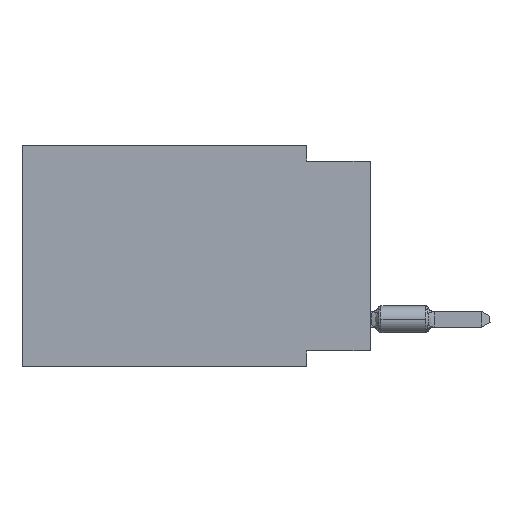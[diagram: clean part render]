
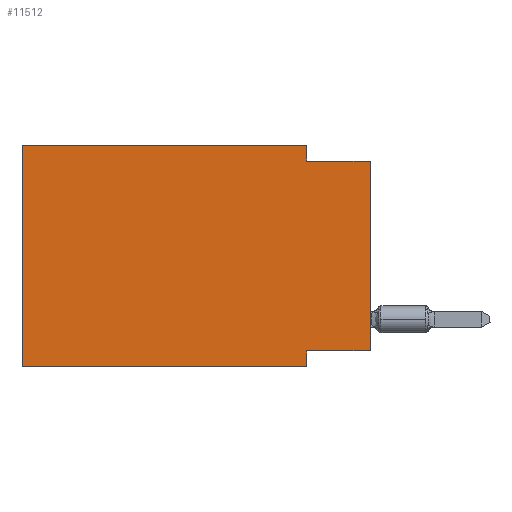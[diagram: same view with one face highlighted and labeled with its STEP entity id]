
A CAD part, left-side view. The second image highlights one B-rep face of the part: STEP entity #11512.
In plain terms, the highlighted planar face has unit normal (-1, 0, 0).
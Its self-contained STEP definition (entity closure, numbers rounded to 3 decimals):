
#978 = ORIENTED_EDGE ( 'NONE', *, *, #32327, .F. ) ;
#1175 = DIRECTION ( 'NONE',  ( 0., 0., -1. ) ) ;
#1207 = CARTESIAN_POINT ( 'NONE',  ( 0., 0., -8.255 ) ) ;
#1449 = CARTESIAN_POINT ( 'NONE',  ( 0., 0., -0.635 ) ) ;
#2517 = CARTESIAN_POINT ( 'NONE',  ( 0., 2.54, -8.255 ) ) ;
#3045 = ORIENTED_EDGE ( 'NONE', *, *, #33190, .F. ) ;
#3414 = VECTOR ( 'NONE', #35923, 1000. ) ;
#5371 = CARTESIAN_POINT ( 'NONE',  ( 0., 13.97, -8.89 ) ) ;
#5551 = EDGE_LOOP ( 'NONE', ( #31347, #14527, #7653, #40815, #9410, #18989, #3045, #978 ) ) ;
#5599 = EDGE_CURVE ( 'NONE', #5946, #6563, #39292, .T. ) ;
#5946 = VERTEX_POINT ( 'NONE', #5371 ) ;
#6563 = VERTEX_POINT ( 'NONE', #30222 ) ;
#6693 = CARTESIAN_POINT ( 'NONE',  ( 0., 13.97, 0. ) ) ;
#7653 = ORIENTED_EDGE ( 'NONE', *, *, #34721, .F. ) ;
#8140 = EDGE_CURVE ( 'NONE', #22937, #24792, #32397, .T. ) ;
#8572 = VECTOR ( 'NONE', #19413, 1000. ) ;
#9410 = ORIENTED_EDGE ( 'NONE', *, *, #16517, .F. ) ;
#9543 = CARTESIAN_POINT ( 'NONE',  ( 0., 13.97, 0. ) ) ;
#9876 = VECTOR ( 'NONE', #12463, 1000. ) ;
#10045 = DIRECTION ( 'NONE',  ( 1., 0., 0. ) ) ;
#10299 = CARTESIAN_POINT ( 'NONE',  ( 0., 2.54, -0.635 ) ) ;
#10809 = CARTESIAN_POINT ( 'NONE',  ( 0., 2.54, 0. ) ) ;
#11512 = ADVANCED_FACE ( 'NONE', ( #43934 ), #30256, .F. ) ;
#11811 = EDGE_CURVE ( 'NONE', #14311, #24792, #18975, .T. ) ;
#12463 = DIRECTION ( 'NONE',  ( 0., -1., 0. ) ) ;
#13838 = EDGE_CURVE ( 'NONE', #37819, #35714, #14929, .T. ) ;
#14311 = VERTEX_POINT ( 'NONE', #1207 ) ;
#14527 = ORIENTED_EDGE ( 'NONE', *, *, #8140, .F. ) ;
#14922 = VECTOR ( 'NONE', #15332, 1000. ) ;
#14929 = LINE ( 'NONE', #38952, #9876 ) ;
#15220 = LINE ( 'NONE', #39028, #25471 ) ;
#15332 = DIRECTION ( 'NONE',  ( 0., -1., 0. ) ) ;
#16517 = EDGE_CURVE ( 'NONE', #5946, #37819, #37134, .T. ) ;
#18211 = LINE ( 'NONE', #39086, #34447 ) ;
#18518 = DIRECTION ( 'NONE',  ( 0., 0., 1. ) ) ;
#18975 = LINE ( 'NONE', #22107, #25456 ) ;
#18989 = ORIENTED_EDGE ( 'NONE', *, *, #5599, .T. ) ;
#19413 = DIRECTION ( 'NONE',  ( 0., 0., 1. ) ) ;
#19772 = CARTESIAN_POINT ( 'NONE',  ( 0., 0., -0.635 ) ) ;
#20135 = DIRECTION ( 'NONE',  ( 0., 0., -1. ) ) ;
#22107 = CARTESIAN_POINT ( 'NONE',  ( 0., 0., 0. ) ) ;
#22451 = CARTESIAN_POINT ( 'NONE',  ( 0., 13.97, -8.89 ) ) ;
#22937 = VERTEX_POINT ( 'NONE', #10299 ) ;
#24792 = VERTEX_POINT ( 'NONE', #19772 ) ;
#25456 = VECTOR ( 'NONE', #18518, 1000. ) ;
#25471 = VECTOR ( 'NONE', #38584, 1000. ) ;
#26122 = VERTEX_POINT ( 'NONE', #2517 ) ;
#29053 = AXIS2_PLACEMENT_3D ( 'NONE', #6693, #10045, #34266 ) ;
#30222 = CARTESIAN_POINT ( 'NONE',  ( 0., 2.54, -8.89 ) ) ;
#30256 = PLANE ( 'NONE',  #29053 ) ;
#31347 = ORIENTED_EDGE ( 'NONE', *, *, #11811, .T. ) ;
#32327 = EDGE_CURVE ( 'NONE', #14311, #26122, #15220, .T. ) ;
#32397 = LINE ( 'NONE', #1449, #14922 ) ;
#33190 = EDGE_CURVE ( 'NONE', #26122, #6563, #18211, .T. ) ;
#34266 = DIRECTION ( 'NONE',  ( 0., 0., -1. ) ) ;
#34447 = VECTOR ( 'NONE', #1175, 1000. ) ;
#34721 = EDGE_CURVE ( 'NONE', #35714, #22937, #40351, .T. ) ;
#35714 = VERTEX_POINT ( 'NONE', #10809 ) ;
#35923 = DIRECTION ( 'NONE',  ( 0., -1., 0. ) ) ;
#37134 = LINE ( 'NONE', #9543, #8572 ) ;
#37819 = VERTEX_POINT ( 'NONE', #40620 ) ;
#38584 = DIRECTION ( 'NONE',  ( 0., 1., 0. ) ) ;
#38952 = CARTESIAN_POINT ( 'NONE',  ( 0., 13.97, 0. ) ) ;
#39028 = CARTESIAN_POINT ( 'NONE',  ( 0., 0., -8.255 ) ) ;
#39086 = CARTESIAN_POINT ( 'NONE',  ( 0., 2.54, -8.89 ) ) ;
#39292 = LINE ( 'NONE', #22451, #3414 ) ;
#40292 = VECTOR ( 'NONE', #20135, 1000. ) ;
#40351 = LINE ( 'NONE', #40785, #40292 ) ;
#40620 = CARTESIAN_POINT ( 'NONE',  ( 0., 13.97, 0. ) ) ;
#40785 = CARTESIAN_POINT ( 'NONE',  ( 0., 2.54, 0. ) ) ;
#40815 = ORIENTED_EDGE ( 'NONE', *, *, #13838, .F. ) ;
#43934 = FACE_OUTER_BOUND ( 'NONE', #5551, .T. ) ;
